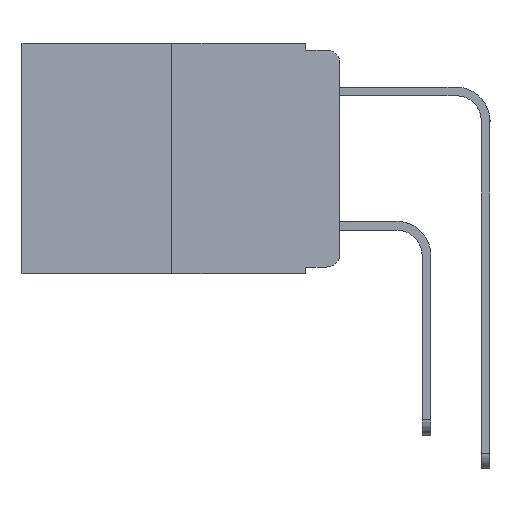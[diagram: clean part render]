
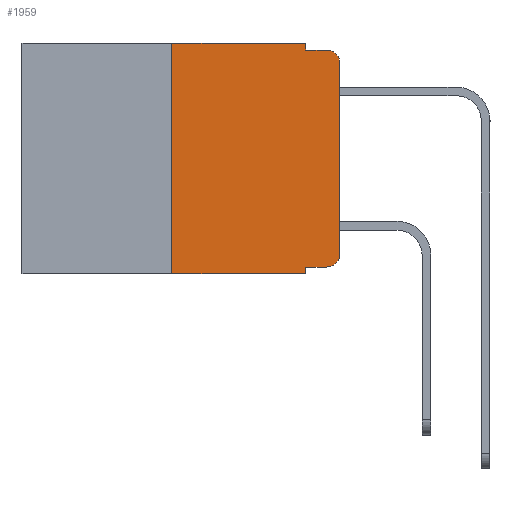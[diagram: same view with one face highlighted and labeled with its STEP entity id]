
A CAD part, left-side view. The second image highlights one B-rep face of the part: STEP entity #1959.
In plain terms, the highlighted planar face has unit normal (-1, 0, 0).
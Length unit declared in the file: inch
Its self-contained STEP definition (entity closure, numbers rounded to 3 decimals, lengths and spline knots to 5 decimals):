
#422 = LINE ( 'NONE', #7990, #5958 ) ;
#540 = VERTEX_POINT ( 'NONE', #13183 ) ;
#852 = DIRECTION ( 'NONE',  ( 0., -1., 0. ) ) ;
#948 = ORIENTED_EDGE ( 'NONE', *, *, #974, .T. ) ;
#974 = EDGE_CURVE ( 'NONE', #1119, #6023, #7345, .T. ) ;
#1119 = VERTEX_POINT ( 'NONE', #4090 ) ;
#1189 = LINE ( 'NONE', #4796, #9713 ) ;
#1202 = CARTESIAN_POINT ( 'NONE',  ( 0., 0., -0.313 ) ) ;
#1860 = EDGE_LOOP ( 'NONE', ( #4775, #5429, #8242, #3617, #12524, #7388, #13457, #5919, #948, #2092 ) ) ;
#1930 = CARTESIAN_POINT ( 'NONE',  ( 0., 0.051, 0. ) ) ;
#1959 = ADVANCED_FACE ( 'NONE', ( #10415 ), #13733, .F. ) ;
#2092 = ORIENTED_EDGE ( 'NONE', *, *, #10468, .T. ) ;
#2593 = CARTESIAN_POINT ( 'NONE',  ( 0., 0.051, -0.333 ) ) ;
#2696 = LINE ( 'NONE', #8590, #5184 ) ;
#2705 = DIRECTION ( 'NONE',  ( 0., 0., -1. ) ) ;
#2830 = DIRECTION ( 'NONE',  ( 0., -1., 0. ) ) ;
#3375 = VECTOR ( 'NONE', #3637, 39.37008 ) ;
#3617 = ORIENTED_EDGE ( 'NONE', *, *, #11707, .F. ) ;
#3637 = DIRECTION ( 'NONE',  ( 0., -1., 0. ) ) ;
#3766 = CARTESIAN_POINT ( 'NONE',  ( 0., 0.02, -0.313 ) ) ;
#4090 = CARTESIAN_POINT ( 'NONE',  ( 0., 0.051, -0.333 ) ) ;
#4302 = EDGE_CURVE ( 'NONE', #540, #7776, #422, .T. ) ;
#4346 = AXIS2_PLACEMENT_3D ( 'NONE', #3766, #11084, #4823 ) ;
#4387 = VERTEX_POINT ( 'NONE', #7372 ) ;
#4707 = CARTESIAN_POINT ( 'NONE',  ( 0., 0.473, 0. ) ) ;
#4775 = ORIENTED_EDGE ( 'NONE', *, *, #5353, .T. ) ;
#4796 = CARTESIAN_POINT ( 'NONE',  ( 0., 0.051, 0. ) ) ;
#4823 = DIRECTION ( 'NONE',  ( 0., 0., -1. ) ) ;
#5158 = DIRECTION ( 'NONE',  ( -1., 0., 0. ) ) ;
#5184 = VECTOR ( 'NONE', #9641, 39.37008 ) ;
#5353 = EDGE_CURVE ( 'NONE', #7745, #5457, #9895, .T. ) ;
#5429 = ORIENTED_EDGE ( 'NONE', *, *, #7450, .T. ) ;
#5457 = VERTEX_POINT ( 'NONE', #11269 ) ;
#5855 = CIRCLE ( 'NONE', #4346, 0.02 ) ;
#5919 = ORIENTED_EDGE ( 'NONE', *, *, #12439, .F. ) ;
#5924 = CARTESIAN_POINT ( 'NONE',  ( 0., 0., 0. ) ) ;
#5958 = VECTOR ( 'NONE', #6680, 39.37008 ) ;
#6023 = VERTEX_POINT ( 'NONE', #11262 ) ;
#6318 = CARTESIAN_POINT ( 'NONE',  ( 0., 0.473, -0.343 ) ) ;
#6445 = AXIS2_PLACEMENT_3D ( 'NONE', #11405, #5158, #12377 ) ;
#6680 = DIRECTION ( 'NONE',  ( 0., 0., 1. ) ) ;
#6757 = CARTESIAN_POINT ( 'NONE',  ( 0., 0.473, 0. ) ) ;
#7106 = DIRECTION ( 'NONE',  ( 0., 0., -1. ) ) ;
#7288 = DIRECTION ( 'NONE',  ( 0., 0., -1. ) ) ;
#7345 = LINE ( 'NONE', #2593, #12181 ) ;
#7372 = CARTESIAN_POINT ( 'NONE',  ( 0., 0.051, -0.01 ) ) ;
#7388 = ORIENTED_EDGE ( 'NONE', *, *, #4302, .F. ) ;
#7450 = EDGE_CURVE ( 'NONE', #5457, #10660, #12369, .T. ) ;
#7745 = VERTEX_POINT ( 'NONE', #1202 ) ;
#7776 = VERTEX_POINT ( 'NONE', #12864 ) ;
#7990 = CARTESIAN_POINT ( 'NONE',  ( 0., 0.25, 0. ) ) ;
#8242 = ORIENTED_EDGE ( 'NONE', *, *, #10261, .F. ) ;
#8277 = LINE ( 'NONE', #12413, #10686 ) ;
#8590 = CARTESIAN_POINT ( 'NONE',  ( 0., 0.051, -0.01 ) ) ;
#8623 = DIRECTION ( 'NONE',  ( 1., 0., 0. ) ) ;
#8771 = EDGE_CURVE ( 'NONE', #540, #12483, #9307, .T. ) ;
#9307 = LINE ( 'NONE', #6318, #11731 ) ;
#9641 = DIRECTION ( 'NONE',  ( 0., -1., 0. ) ) ;
#9713 = VECTOR ( 'NONE', #2705, 39.37008 ) ;
#9729 = EDGE_CURVE ( 'NONE', #7776, #12428, #13395, .T. ) ;
#9895 = LINE ( 'NONE', #5924, #12284 ) ;
#10261 = EDGE_CURVE ( 'NONE', #4387, #10660, #2696, .T. ) ;
#10415 = FACE_OUTER_BOUND ( 'NONE', #1860, .T. ) ;
#10433 = CARTESIAN_POINT ( 'NONE',  ( 0., 0.051, -0.343 ) ) ;
#10468 = EDGE_CURVE ( 'NONE', #6023, #7745, #5855, .T. ) ;
#10471 = CARTESIAN_POINT ( 'NONE',  ( 0., 0.02, -0.01 ) ) ;
#10660 = VERTEX_POINT ( 'NONE', #10471 ) ;
#10686 = VECTOR ( 'NONE', #7288, 39.37008 ) ;
#11084 = DIRECTION ( 'NONE',  ( -1., 0., 0. ) ) ;
#11262 = CARTESIAN_POINT ( 'NONE',  ( 0., 0.02, -0.333 ) ) ;
#11269 = CARTESIAN_POINT ( 'NONE',  ( 0., 0., -0.03 ) ) ;
#11405 = CARTESIAN_POINT ( 'NONE',  ( 0., 0.02, -0.03 ) ) ;
#11707 = EDGE_CURVE ( 'NONE', #12428, #4387, #1189, .T. ) ;
#11731 = VECTOR ( 'NONE', #852, 39.37008 ) ;
#12181 = VECTOR ( 'NONE', #2830, 39.37008 ) ;
#12284 = VECTOR ( 'NONE', #13123, 39.37008 ) ;
#12369 = CIRCLE ( 'NONE', #6445, 0.02 ) ;
#12377 = DIRECTION ( 'NONE',  ( 0., 0., -1. ) ) ;
#12413 = CARTESIAN_POINT ( 'NONE',  ( 0., 0.051, 0. ) ) ;
#12428 = VERTEX_POINT ( 'NONE', #1930 ) ;
#12439 = EDGE_CURVE ( 'NONE', #1119, #12483, #8277, .T. ) ;
#12444 = AXIS2_PLACEMENT_3D ( 'NONE', #6757, #8623, #7106 ) ;
#12483 = VERTEX_POINT ( 'NONE', #10433 ) ;
#12524 = ORIENTED_EDGE ( 'NONE', *, *, #9729, .F. ) ;
#12864 = CARTESIAN_POINT ( 'NONE',  ( 0., 0.25, 0. ) ) ;
#13123 = DIRECTION ( 'NONE',  ( 0., 0., 1. ) ) ;
#13183 = CARTESIAN_POINT ( 'NONE',  ( 0., 0.25, -0.343 ) ) ;
#13395 = LINE ( 'NONE', #4707, #3375 ) ;
#13457 = ORIENTED_EDGE ( 'NONE', *, *, #8771, .T. ) ;
#13733 = PLANE ( 'NONE',  #12444 ) ;
